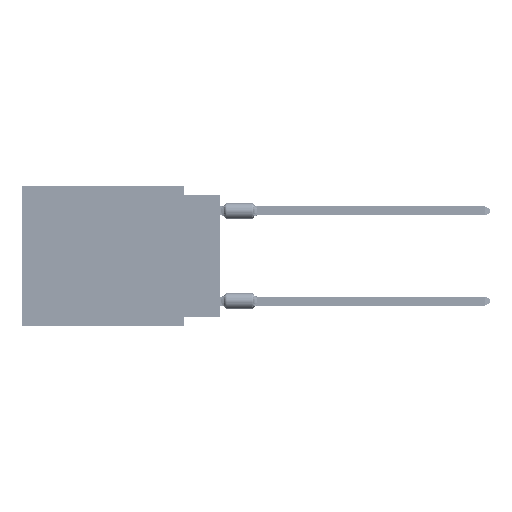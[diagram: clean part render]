
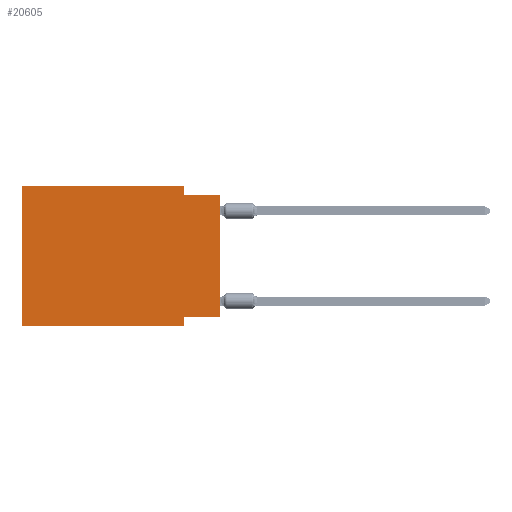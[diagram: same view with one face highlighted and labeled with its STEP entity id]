
A CAD part, left-side view. The second image highlights one B-rep face of the part: STEP entity #20605.
In plain terms, the highlighted planar face has unit normal (-1, 0, 0).
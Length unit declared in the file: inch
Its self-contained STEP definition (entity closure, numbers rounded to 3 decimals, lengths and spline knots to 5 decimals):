
#1549 = DIRECTION ( 'NONE',  ( 0., -1., 0. ) ) ;
#2662 = LINE ( 'NONE', #15072, #21415 ) ;
#2998 = CARTESIAN_POINT ( 'NONE',  ( 0., 0.55, 0. ) ) ;
#3133 = VECTOR ( 'NONE', #1549, 39.37008 ) ;
#3177 = VERTEX_POINT ( 'NONE', #69634 ) ;
#3432 = DIRECTION ( 'NONE',  ( 1., 0., 0. ) ) ;
#6656 = VERTEX_POINT ( 'NONE', #82722 ) ;
#8455 = VERTEX_POINT ( 'NONE', #34777 ) ;
#9645 = CARTESIAN_POINT ( 'NONE',  ( 0., 0., 0. ) ) ;
#10121 = DIRECTION ( 'NONE',  ( 0., 0., -1. ) ) ;
#11540 = CARTESIAN_POINT ( 'NONE',  ( 0., 0., -0.025 ) ) ;
#13650 = ORIENTED_EDGE ( 'NONE', *, *, #86654, .F. ) ;
#13812 = CARTESIAN_POINT ( 'NONE',  ( 0., 0.55, 0. ) ) ;
#14240 = CARTESIAN_POINT ( 'NONE',  ( 0., 0.1, 0. ) ) ;
#14994 = DIRECTION ( 'NONE',  ( 0., 0., 1. ) ) ;
#15072 = CARTESIAN_POINT ( 'NONE',  ( 0., 0., -0.365 ) ) ;
#15457 = EDGE_CURVE ( 'NONE', #8455, #50935, #70658, .T. ) ;
#15500 = DIRECTION ( 'NONE',  ( 0., 1., 0. ) ) ;
#17152 = LINE ( 'NONE', #58210, #42363 ) ;
#18462 = DIRECTION ( 'NONE',  ( 0., 0., 1. ) ) ;
#20191 = EDGE_CURVE ( 'NONE', #74902, #3177, #2662, .T. ) ;
#20605 = ADVANCED_FACE ( 'NONE', ( #37007 ), #50698, .F. ) ;
#20980 = CARTESIAN_POINT ( 'NONE',  ( 0., 0.55, 0. ) ) ;
#21415 = VECTOR ( 'NONE', #15500, 39.37008 ) ;
#22954 = ORIENTED_EDGE ( 'NONE', *, *, #63989, .F. ) ;
#23368 = CARTESIAN_POINT ( 'NONE',  ( 0., 0.1, 0. ) ) ;
#26793 = VECTOR ( 'NONE', #37105, 39.37008 ) ;
#29699 = CARTESIAN_POINT ( 'NONE',  ( 0., 0.1, -0.39 ) ) ;
#32564 = VERTEX_POINT ( 'NONE', #78197 ) ;
#34777 = CARTESIAN_POINT ( 'NONE',  ( 0., 0.55, -0.39 ) ) ;
#37007 = FACE_OUTER_BOUND ( 'NONE', #85296, .T. ) ;
#37105 = DIRECTION ( 'NONE',  ( 0., -1., 0. ) ) ;
#37765 = VECTOR ( 'NONE', #10121, 39.37008 ) ;
#42363 = VECTOR ( 'NONE', #18462, 39.37008 ) ;
#43203 = DIRECTION ( 'NONE',  ( 0., 0., -1. ) ) ;
#44603 = CARTESIAN_POINT ( 'NONE',  ( 0., 0.55, -0.39 ) ) ;
#47228 = ORIENTED_EDGE ( 'NONE', *, *, #20191, .F. ) ;
#50698 = PLANE ( 'NONE',  #69418 ) ;
#50935 = VERTEX_POINT ( 'NONE', #29699 ) ;
#53789 = VECTOR ( 'NONE', #75241, 39.37008 ) ;
#54925 = VECTOR ( 'NONE', #14994, 39.37008 ) ;
#54961 = LINE ( 'NONE', #68185, #53789 ) ;
#55212 = LINE ( 'NONE', #23368, #37765 ) ;
#57007 = EDGE_CURVE ( 'NONE', #59785, #32564, #55212, .T. ) ;
#58210 = CARTESIAN_POINT ( 'NONE',  ( 0., 0.55, 0. ) ) ;
#59785 = VERTEX_POINT ( 'NONE', #14240 ) ;
#61350 = ORIENTED_EDGE ( 'NONE', *, *, #72596, .T. ) ;
#61472 = VECTOR ( 'NONE', #72010, 39.37008 ) ;
#61582 = LINE ( 'NONE', #20980, #3133 ) ;
#63062 = LINE ( 'NONE', #9645, #54925 ) ;
#63989 = EDGE_CURVE ( 'NONE', #77777, #59785, #61582, .T. ) ;
#65494 = CARTESIAN_POINT ( 'NONE',  ( 0., 0., -0.365 ) ) ;
#65734 = ORIENTED_EDGE ( 'NONE', *, *, #57007, .F. ) ;
#67267 = ORIENTED_EDGE ( 'NONE', *, *, #76331, .F. ) ;
#68185 = CARTESIAN_POINT ( 'NONE',  ( 0., 0.1, -0.39 ) ) ;
#69418 = AXIS2_PLACEMENT_3D ( 'NONE', #2998, #3432, #43203 ) ;
#69634 = CARTESIAN_POINT ( 'NONE',  ( 0., 0.1, -0.365 ) ) ;
#70658 = LINE ( 'NONE', #44603, #26793 ) ;
#70705 = LINE ( 'NONE', #11540, #61472 ) ;
#71529 = ORIENTED_EDGE ( 'NONE', *, *, #15457, .T. ) ;
#72010 = DIRECTION ( 'NONE',  ( 0., -1., 0. ) ) ;
#72596 = EDGE_CURVE ( 'NONE', #74902, #6656, #63062, .T. ) ;
#74902 = VERTEX_POINT ( 'NONE', #65494 ) ;
#75241 = DIRECTION ( 'NONE',  ( 0., 0., -1. ) ) ;
#75595 = EDGE_CURVE ( 'NONE', #8455, #77777, #17152, .T. ) ;
#76331 = EDGE_CURVE ( 'NONE', #3177, #50935, #54961, .T. ) ;
#77223 = ORIENTED_EDGE ( 'NONE', *, *, #75595, .F. ) ;
#77777 = VERTEX_POINT ( 'NONE', #13812 ) ;
#78197 = CARTESIAN_POINT ( 'NONE',  ( 0., 0.1, -0.025 ) ) ;
#82722 = CARTESIAN_POINT ( 'NONE',  ( 0., 0., -0.025 ) ) ;
#85296 = EDGE_LOOP ( 'NONE', ( #61350, #13650, #65734, #22954, #77223, #71529, #67267, #47228 ) ) ;
#86654 = EDGE_CURVE ( 'NONE', #32564, #6656, #70705, .T. ) ;
